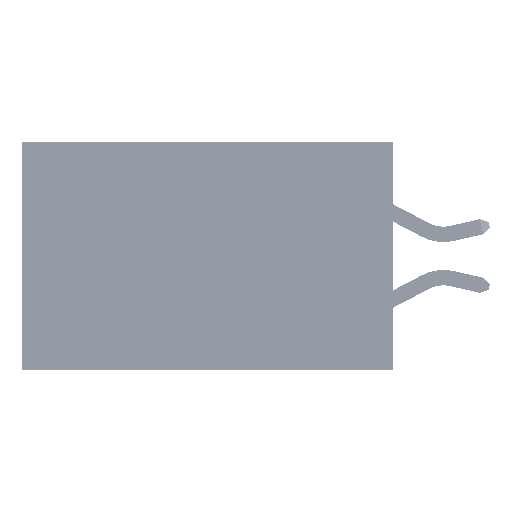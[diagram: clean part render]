
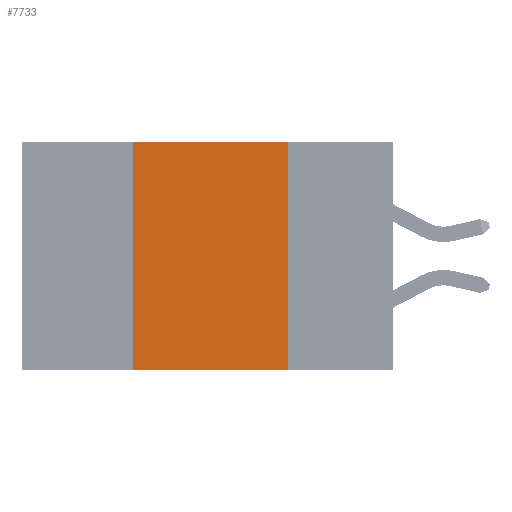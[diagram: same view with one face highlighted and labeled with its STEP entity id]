
A CAD part, left-side view. The second image highlights one B-rep face of the part: STEP entity #7733.
In plain terms, the highlighted planar face has unit normal (-1, 0, 0).
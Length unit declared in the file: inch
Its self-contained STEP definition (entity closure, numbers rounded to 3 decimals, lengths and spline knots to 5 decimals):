
#191 = LINE ( 'NONE', #40242, #41239 ) ;
#2621 = DIRECTION ( 'NONE',  ( 0., 0., -1. ) ) ;
#2797 = LINE ( 'NONE', #23800, #45034 ) ;
#3531 = EDGE_LOOP ( 'NONE', ( #45480, #10832, #13364, #24585 ) ) ;
#3968 = DIRECTION ( 'NONE',  ( 0., -1., 0. ) ) ;
#5200 = EDGE_CURVE ( 'NONE', #30179, #42629, #191, .T. ) ;
#5461 = CARTESIAN_POINT ( 'NONE',  ( 0., 0.17, 0. ) ) ;
#7733 = ADVANCED_FACE ( 'NONE', ( #37371 ), #51272, .F. ) ;
#10832 = ORIENTED_EDGE ( 'NONE', *, *, #30968, .F. ) ;
#12037 = DIRECTION ( 'NONE',  ( 0., 0., -1. ) ) ;
#13364 = ORIENTED_EDGE ( 'NONE', *, *, #30933, .F. ) ;
#14342 = VERTEX_POINT ( 'NONE', #50390 ) ;
#15192 = CARTESIAN_POINT ( 'NONE',  ( 0., 0.42, -0.37 ) ) ;
#19394 = VECTOR ( 'NONE', #2621, 39.37008 ) ;
#20794 = CARTESIAN_POINT ( 'NONE',  ( 0., 0.6, 0. ) ) ;
#22871 = LINE ( 'NONE', #20794, #43773 ) ;
#23800 = CARTESIAN_POINT ( 'NONE',  ( 0., 0.42, 0. ) ) ;
#24585 = ORIENTED_EDGE ( 'NONE', *, *, #5200, .T. ) ;
#24611 = DIRECTION ( 'NONE',  ( 0., -1., 0. ) ) ;
#26327 = AXIS2_PLACEMENT_3D ( 'NONE', #46777, #35744, #12037 ) ;
#26554 = CARTESIAN_POINT ( 'NONE',  ( 0., 0.17, 0. ) ) ;
#30179 = VERTEX_POINT ( 'NONE', #15192 ) ;
#30933 = EDGE_CURVE ( 'NONE', #30179, #14342, #2797, .T. ) ;
#30968 = EDGE_CURVE ( 'NONE', #14342, #50120, #22871, .T. ) ;
#35744 = DIRECTION ( 'NONE',  ( 1., 0., 0. ) ) ;
#37371 = FACE_OUTER_BOUND ( 'NONE', #3531, .T. ) ;
#37887 = LINE ( 'NONE', #26554, #19394 ) ;
#40242 = CARTESIAN_POINT ( 'NONE',  ( 0., 0.6, -0.37 ) ) ;
#41239 = VECTOR ( 'NONE', #24611, 39.37008 ) ;
#42629 = VERTEX_POINT ( 'NONE', #48027 ) ;
#43773 = VECTOR ( 'NONE', #3968, 39.37008 ) ;
#45034 = VECTOR ( 'NONE', #51189, 39.37008 ) ;
#45480 = ORIENTED_EDGE ( 'NONE', *, *, #45798, .F. ) ;
#45798 = EDGE_CURVE ( 'NONE', #50120, #42629, #37887, .T. ) ;
#46777 = CARTESIAN_POINT ( 'NONE',  ( 0., 0.6, 0. ) ) ;
#48027 = CARTESIAN_POINT ( 'NONE',  ( 0., 0.17, -0.37 ) ) ;
#50120 = VERTEX_POINT ( 'NONE', #5461 ) ;
#50390 = CARTESIAN_POINT ( 'NONE',  ( 0., 0.42, 0. ) ) ;
#51189 = DIRECTION ( 'NONE',  ( 0., 0., 1. ) ) ;
#51272 = PLANE ( 'NONE',  #26327 ) ;
